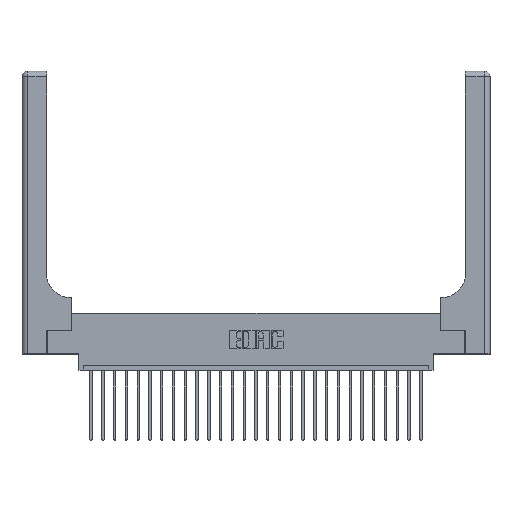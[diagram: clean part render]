
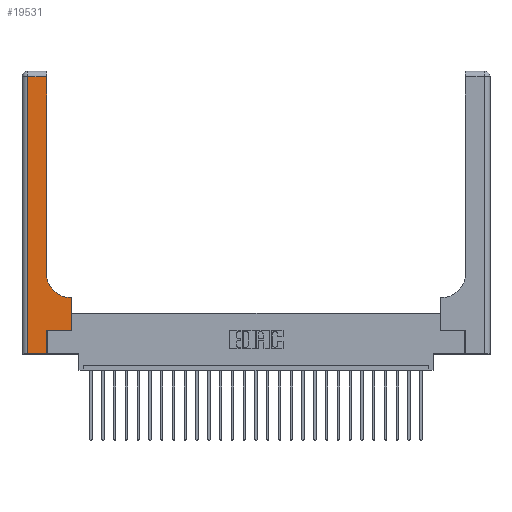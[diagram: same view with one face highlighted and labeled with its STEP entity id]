
A CAD part, top view. The second image highlights one B-rep face of the part: STEP entity #19531.
In plain terms, the highlighted planar face has unit normal (0, 0, 1).
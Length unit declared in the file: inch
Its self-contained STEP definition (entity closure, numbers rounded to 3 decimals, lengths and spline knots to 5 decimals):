
#241 = EDGE_CURVE ( 'NONE', #5889, #10527, #22157, .T. ) ;
#441 = CARTESIAN_POINT ( 'NONE',  ( 0.51, 0.6, 0.37 ) ) ;
#1242 = ORIENTED_EDGE ( 'NONE', *, *, #15777, .T. ) ;
#1987 = ORIENTED_EDGE ( 'NONE', *, *, #7994, .T. ) ;
#2271 = EDGE_CURVE ( 'NONE', #8239, #3873, #4480, .T. ) ;
#2982 = DIRECTION ( 'NONE',  ( 0., 0., -1. ) ) ;
#3206 = VECTOR ( 'NONE', #20215, 39.37008 ) ;
#3873 = VERTEX_POINT ( 'NONE', #21852 ) ;
#4410 = EDGE_CURVE ( 'NONE', #10358, #8239, #11071, .T. ) ;
#4480 = LINE ( 'NONE', #8735, #3206 ) ;
#4819 = CARTESIAN_POINT ( 'NONE',  ( 0.51, 0.85, 0.37 ) ) ;
#5285 = EDGE_CURVE ( 'NONE', #3873, #5742, #10875, .T. ) ;
#5440 = VECTOR ( 'NONE', #12815, 39.37008 ) ;
#5742 = VERTEX_POINT ( 'NONE', #16303 ) ;
#5795 = CARTESIAN_POINT ( 'NONE',  ( 0.528, 0.6, 0.37 ) ) ;
#5831 = ORIENTED_EDGE ( 'NONE', *, *, #22553, .T. ) ;
#5889 = VERTEX_POINT ( 'NONE', #441 ) ;
#6151 = LINE ( 'NONE', #17768, #22462 ) ;
#7018 = VECTOR ( 'NONE', #22592, 39.37008 ) ;
#7271 = VERTEX_POINT ( 'NONE', #15415 ) ;
#7712 = DIRECTION ( 'NONE',  ( 0., 1., 0. ) ) ;
#7994 = EDGE_CURVE ( 'NONE', #7271, #10358, #20777, .T. ) ;
#8209 = CARTESIAN_POINT ( 'NONE',  ( 0.528, 0.25, 0.37 ) ) ;
#8239 = VERTEX_POINT ( 'NONE', #17032 ) ;
#8735 = CARTESIAN_POINT ( 'NONE',  ( 0.265, 0., 0.37 ) ) ;
#9635 = AXIS2_PLACEMENT_3D ( 'NONE', #24914, #2982, #18709 ) ;
#10147 = LINE ( 'NONE', #8209, #24579 ) ;
#10271 = CARTESIAN_POINT ( 'NONE',  ( 0.26, 0.6, 0.37 ) ) ;
#10358 = VERTEX_POINT ( 'NONE', #16620 ) ;
#10527 = VERTEX_POINT ( 'NONE', #21772 ) ;
#10875 = LINE ( 'NONE', #22381, #5440 ) ;
#10901 = ORIENTED_EDGE ( 'NONE', *, *, #2271, .T. ) ;
#11034 = AXIS2_PLACEMENT_3D ( 'NONE', #4819, #18614, #15007 ) ;
#11071 = LINE ( 'NONE', #14699, #7018 ) ;
#11597 = VECTOR ( 'NONE', #15654, 39.37008 ) ;
#12639 = ORIENTED_EDGE ( 'NONE', *, *, #19818, .T. ) ;
#12815 = DIRECTION ( 'NONE',  ( 1., 0., 0. ) ) ;
#13074 = ORIENTED_EDGE ( 'NONE', *, *, #241, .T. ) ;
#14699 = CARTESIAN_POINT ( 'NONE',  ( 0., 0., 0.37 ) ) ;
#15007 = DIRECTION ( 'NONE',  ( 1., 0., 0. ) ) ;
#15071 = EDGE_LOOP ( 'NONE', ( #1242, #5831, #1987, #23910, #10901, #23565, #15990, #12639, #13074 ) ) ;
#15292 = CARTESIAN_POINT ( 'NONE',  ( 0.26, 2.94, 0.37 ) ) ;
#15415 = CARTESIAN_POINT ( 'NONE',  ( 0.06, 2.94, 0.37 ) ) ;
#15654 = DIRECTION ( 'NONE',  ( -1., 0., 0. ) ) ;
#15777 = EDGE_CURVE ( 'NONE', #10527, #16462, #6151, .T. ) ;
#15990 = ORIENTED_EDGE ( 'NONE', *, *, #24863, .T. ) ;
#16303 = CARTESIAN_POINT ( 'NONE',  ( 0.528, 0.25, 0.37 ) ) ;
#16462 = VERTEX_POINT ( 'NONE', #15292 ) ;
#16508 = FACE_OUTER_BOUND ( 'NONE', #15071, .T. ) ;
#16620 = CARTESIAN_POINT ( 'NONE',  ( 0.06, 0., 0.37 ) ) ;
#16645 = DIRECTION ( 'NONE',  ( 0., -1., 0. ) ) ;
#17032 = CARTESIAN_POINT ( 'NONE',  ( 0.265, 0., 0.37 ) ) ;
#17578 = CARTESIAN_POINT ( 'NONE',  ( 0., 2.94, 0.37 ) ) ;
#17672 = VECTOR ( 'NONE', #16645, 39.37008 ) ;
#17768 = CARTESIAN_POINT ( 'NONE',  ( 0.26, 3., 0.37 ) ) ;
#17905 = DIRECTION ( 'NONE',  ( -1., 0., 0. ) ) ;
#18614 = DIRECTION ( 'NONE',  ( 0., 0., -1. ) ) ;
#18709 = DIRECTION ( 'NONE',  ( -1., 0., 0. ) ) ;
#19531 = ADVANCED_FACE ( 'NONE', ( #16508 ), #22469, .F. ) ;
#19818 = EDGE_CURVE ( 'NONE', #23174, #5889, #23982, .T. ) ;
#20215 = DIRECTION ( 'NONE',  ( 0., 1., 0. ) ) ;
#20777 = LINE ( 'NONE', #24547, #17672 ) ;
#21453 = LINE ( 'NONE', #17578, #11597 ) ;
#21600 = VECTOR ( 'NONE', #17905, 39.37008 ) ;
#21772 = CARTESIAN_POINT ( 'NONE',  ( 0.26, 0.85, 0.37 ) ) ;
#21852 = CARTESIAN_POINT ( 'NONE',  ( 0.265, 0.25, 0.37 ) ) ;
#22157 = CIRCLE ( 'NONE', #11034, 0.25 ) ;
#22381 = CARTESIAN_POINT ( 'NONE',  ( 0.265, 0.25, 0.37 ) ) ;
#22462 = VECTOR ( 'NONE', #7712, 39.37008 ) ;
#22469 = PLANE ( 'NONE',  #9635 ) ;
#22553 = EDGE_CURVE ( 'NONE', #16462, #7271, #21453, .T. ) ;
#22592 = DIRECTION ( 'NONE',  ( 1., 0., 0. ) ) ;
#23174 = VERTEX_POINT ( 'NONE', #5795 ) ;
#23565 = ORIENTED_EDGE ( 'NONE', *, *, #5285, .T. ) ;
#23910 = ORIENTED_EDGE ( 'NONE', *, *, #4410, .T. ) ;
#23982 = LINE ( 'NONE', #10271, #21600 ) ;
#24115 = DIRECTION ( 'NONE',  ( 0., 1., 0. ) ) ;
#24547 = CARTESIAN_POINT ( 'NONE',  ( 0.06, 3., 0.37 ) ) ;
#24579 = VECTOR ( 'NONE', #24115, 39.37008 ) ;
#24863 = EDGE_CURVE ( 'NONE', #5742, #23174, #10147, .T. ) ;
#24914 = CARTESIAN_POINT ( 'NONE',  ( 0., 3., 0.37 ) ) ;
